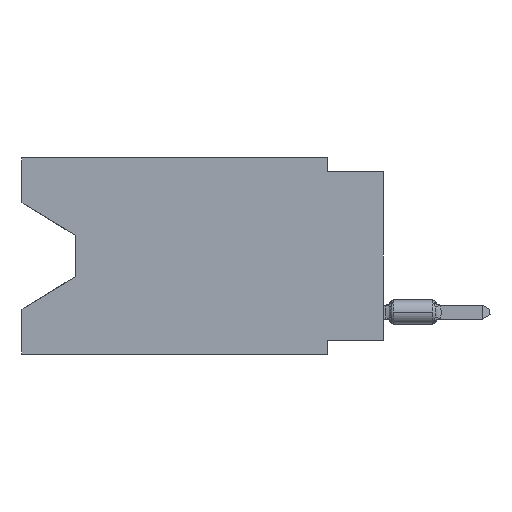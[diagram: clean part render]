
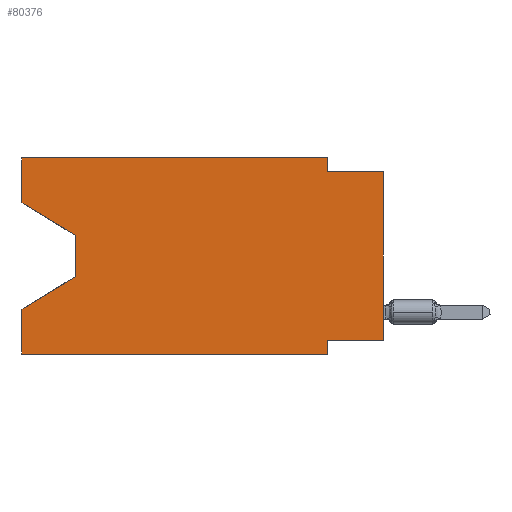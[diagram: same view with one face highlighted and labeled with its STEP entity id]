
A CAD part, left-side view. The second image highlights one B-rep face of the part: STEP entity #80376.
In plain terms, the highlighted planar face has unit normal (-1, 0, 0).
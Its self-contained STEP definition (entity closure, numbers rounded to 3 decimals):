
#230 = FACE_OUTER_BOUND ( 'NONE', #42852, .T. ) ;
#648 = VERTEX_POINT ( 'NONE', #17247 ) ;
#1410 = ORIENTED_EDGE ( 'NONE', *, *, #72749, .T. ) ;
#2326 = EDGE_CURVE ( 'NONE', #29284, #7870, #74034, .T. ) ;
#2940 = VERTEX_POINT ( 'NONE', #41226 ) ;
#3366 = VECTOR ( 'NONE', #18330, 1000. ) ;
#3480 = VECTOR ( 'NONE', #5987, 1000. ) ;
#4113 = EDGE_CURVE ( 'NONE', #48146, #48931, #6757, .T. ) ;
#5520 = VERTEX_POINT ( 'NONE', #62293 ) ;
#5651 = VECTOR ( 'NONE', #79090, 1000. ) ;
#5852 = CARTESIAN_POINT ( 'NONE',  ( 0., 16.383, -6.852 ) ) ;
#5987 = DIRECTION ( 'NONE',  ( 0., -1., 0. ) ) ;
#6078 = EDGE_CURVE ( 'NONE', #5520, #7870, #24084, .T. ) ;
#6757 = LINE ( 'NONE', #45093, #53645 ) ;
#7870 = VERTEX_POINT ( 'NONE', #5852 ) ;
#11215 = VECTOR ( 'NONE', #73672, 1000. ) ;
#11336 = CARTESIAN_POINT ( 'NONE',  ( 0., 16.383, -8.89 ) ) ;
#11381 = DIRECTION ( 'NONE',  ( 0., 0.855, -0.519 ) ) ;
#11846 = ORIENTED_EDGE ( 'NONE', *, *, #13296, .F. ) ;
#13296 = EDGE_CURVE ( 'NONE', #39923, #648, #47779, .T. ) ;
#14860 = VECTOR ( 'NONE', #35373, 1000. ) ;
#14933 = CARTESIAN_POINT ( 'NONE',  ( 0., 0., 0. ) ) ;
#17247 = CARTESIAN_POINT ( 'NONE',  ( 0., 2.54, -8.89 ) ) ;
#17508 = LINE ( 'NONE', #36072, #3366 ) ;
#17541 = DIRECTION ( 'NONE',  ( 1., 0., 0. ) ) ;
#18330 = DIRECTION ( 'NONE',  ( 0., -0.855, -0.519 ) ) ;
#19013 = EDGE_CURVE ( 'NONE', #48931, #64342, #55932, .T. ) ;
#22858 = DIRECTION ( 'NONE',  ( 0., 0., 1. ) ) ;
#22947 = CARTESIAN_POINT ( 'NONE',  ( 0., 13.97, -5.385 ) ) ;
#24084 = LINE ( 'NONE', #36454, #44635 ) ;
#24561 = PLANE ( 'NONE',  #49672 ) ;
#28030 = DIRECTION ( 'NONE',  ( 0., 0., -1. ) ) ;
#28213 = ORIENTED_EDGE ( 'NONE', *, *, #2326, .T. ) ;
#28975 = EDGE_CURVE ( 'NONE', #64342, #29356, #56874, .T. ) ;
#29284 = VERTEX_POINT ( 'NONE', #57599 ) ;
#29356 = VERTEX_POINT ( 'NONE', #43996 ) ;
#30373 = ORIENTED_EDGE ( 'NONE', *, *, #71093, .F. ) ;
#30646 = ORIENTED_EDGE ( 'NONE', *, *, #66599, .F. ) ;
#30810 = CARTESIAN_POINT ( 'NONE',  ( 0., 16.383, 0. ) ) ;
#32391 = VECTOR ( 'NONE', #38327, 1000. ) ;
#34336 = CARTESIAN_POINT ( 'NONE',  ( 0., 16.383, 0. ) ) ;
#34567 = LINE ( 'NONE', #42359, #11215 ) ;
#35373 = DIRECTION ( 'NONE',  ( 0., -1., 0. ) ) ;
#36072 = CARTESIAN_POINT ( 'NONE',  ( 0., 16.383, -2.038 ) ) ;
#36454 = CARTESIAN_POINT ( 'NONE',  ( 0., 16.383, 0. ) ) ;
#37550 = ORIENTED_EDGE ( 'NONE', *, *, #19013, .F. ) ;
#37671 = CARTESIAN_POINT ( 'NONE',  ( 0., 0., -8.255 ) ) ;
#38279 = VERTEX_POINT ( 'NONE', #37671 ) ;
#38327 = DIRECTION ( 'NONE',  ( 0., 0., -1. ) ) ;
#39923 = VERTEX_POINT ( 'NONE', #50180 ) ;
#39975 = CARTESIAN_POINT ( 'NONE',  ( 0., 2.54, -8.89 ) ) ;
#40551 = CARTESIAN_POINT ( 'NONE',  ( 0., 0., -0.635 ) ) ;
#41226 = CARTESIAN_POINT ( 'NONE',  ( 0., 13.97, -3.505 ) ) ;
#42249 = CARTESIAN_POINT ( 'NONE',  ( 0., 13.97, -3.505 ) ) ;
#42359 = CARTESIAN_POINT ( 'NONE',  ( 0., 0., -8.255 ) ) ;
#42694 = DIRECTION ( 'NONE',  ( 0., 0., -1. ) ) ;
#42852 = EDGE_LOOP ( 'NONE', ( #78539, #73727, #28213, #71019, #1410, #11846, #30373, #66331, #30646, #79797, #37550, #75073 ) ) ;
#43996 = CARTESIAN_POINT ( 'NONE',  ( 0., 2.54, -0.635 ) ) ;
#44589 = EDGE_CURVE ( 'NONE', #2940, #29284, #60800, .T. ) ;
#44635 = VECTOR ( 'NONE', #22858, 1000. ) ;
#45093 = CARTESIAN_POINT ( 'NONE',  ( 0., 16.383, 0. ) ) ;
#45539 = VECTOR ( 'NONE', #11381, 1000. ) ;
#47779 = LINE ( 'NONE', #39975, #61663 ) ;
#48146 = VERTEX_POINT ( 'NONE', #65946 ) ;
#48931 = VERTEX_POINT ( 'NONE', #34336 ) ;
#49672 = AXIS2_PLACEMENT_3D ( 'NONE', #74832, #17541, #42694 ) ;
#50180 = CARTESIAN_POINT ( 'NONE',  ( 0., 2.54, -8.255 ) ) ;
#50692 = CARTESIAN_POINT ( 'NONE',  ( 0., 2.54, 0. ) ) ;
#52693 = EDGE_CURVE ( 'NONE', #38279, #76611, #64416, .T. ) ;
#53645 = VECTOR ( 'NONE', #68986, 1000. ) ;
#53953 = LINE ( 'NONE', #58945, #5651 ) ;
#55244 = VECTOR ( 'NONE', #71800, 1000. ) ;
#55932 = LINE ( 'NONE', #30810, #14860 ) ;
#56874 = LINE ( 'NONE', #50692, #32391 ) ;
#57599 = CARTESIAN_POINT ( 'NONE',  ( 0., 13.97, -5.385 ) ) ;
#58945 = CARTESIAN_POINT ( 'NONE',  ( 0., 0., -0.635 ) ) ;
#60800 = LINE ( 'NONE', #42249, #69421 ) ;
#61663 = VECTOR ( 'NONE', #28030, 1000. ) ;
#62293 = CARTESIAN_POINT ( 'NONE',  ( 0., 16.383, -8.89 ) ) ;
#63264 = LINE ( 'NONE', #11336, #3480 ) ;
#64342 = VERTEX_POINT ( 'NONE', #69018 ) ;
#64416 = LINE ( 'NONE', #14933, #55244 ) ;
#65946 = CARTESIAN_POINT ( 'NONE',  ( 0., 16.383, -2.038 ) ) ;
#66331 = ORIENTED_EDGE ( 'NONE', *, *, #52693, .T. ) ;
#66599 = EDGE_CURVE ( 'NONE', #29356, #76611, #53953, .T. ) ;
#68986 = DIRECTION ( 'NONE',  ( 0., 0., 1. ) ) ;
#69018 = CARTESIAN_POINT ( 'NONE',  ( 0., 2.54, 0. ) ) ;
#69421 = VECTOR ( 'NONE', #72357, 1000. ) ;
#71019 = ORIENTED_EDGE ( 'NONE', *, *, #6078, .F. ) ;
#71093 = EDGE_CURVE ( 'NONE', #38279, #39923, #34567, .T. ) ;
#71611 = EDGE_CURVE ( 'NONE', #48146, #2940, #17508, .T. ) ;
#71800 = DIRECTION ( 'NONE',  ( 0., 0., 1. ) ) ;
#72357 = DIRECTION ( 'NONE',  ( 0., 0., -1. ) ) ;
#72749 = EDGE_CURVE ( 'NONE', #5520, #648, #63264, .T. ) ;
#73672 = DIRECTION ( 'NONE',  ( 0., 1., 0. ) ) ;
#73727 = ORIENTED_EDGE ( 'NONE', *, *, #44589, .T. ) ;
#74034 = LINE ( 'NONE', #22947, #45539 ) ;
#74832 = CARTESIAN_POINT ( 'NONE',  ( 0., 16.383, 0. ) ) ;
#75073 = ORIENTED_EDGE ( 'NONE', *, *, #4113, .F. ) ;
#76611 = VERTEX_POINT ( 'NONE', #40551 ) ;
#78539 = ORIENTED_EDGE ( 'NONE', *, *, #71611, .T. ) ;
#79090 = DIRECTION ( 'NONE',  ( 0., -1., 0. ) ) ;
#79797 = ORIENTED_EDGE ( 'NONE', *, *, #28975, .F. ) ;
#80376 = ADVANCED_FACE ( 'NONE', ( #230 ), #24561, .F. ) ;
